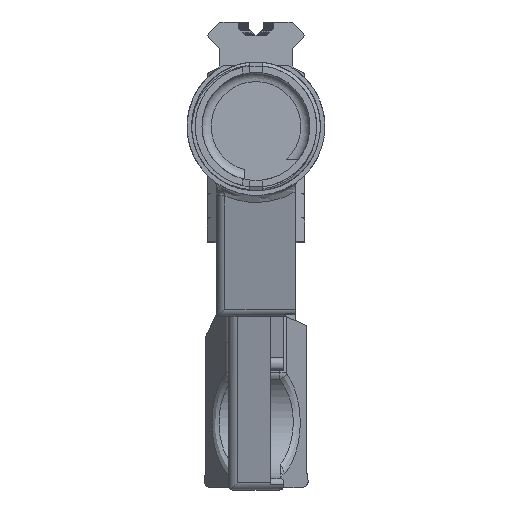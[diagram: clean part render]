
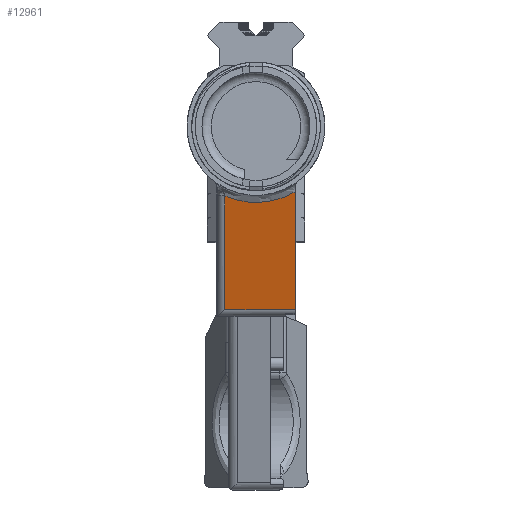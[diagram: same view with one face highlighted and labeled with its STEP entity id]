
A CAD part, front view. The second image highlights one B-rep face of the part: STEP entity #12961.
In plain terms, the highlighted planar face has unit normal (0, -0.972, -0.236).
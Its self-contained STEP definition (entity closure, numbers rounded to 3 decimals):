
#182=ELLIPSE('',#13804,17.416,16.925);
#598=PLANE('',#13806);
#1279=FACE_OUTER_BOUND('',#1988,.T.);
#1988=EDGE_LOOP('',(#11816,#11817,#11818,#11819));
#3605=LINE('',#23635,#4961);
#3606=LINE('',#23648,#4962);
#3612=LINE('',#23712,#4968);
#4961=VECTOR('',#16016,10.);
#4962=VECTOR('',#16019,10.);
#4968=VECTOR('',#16039,10.);
#6250=VERTEX_POINT('',#23632);
#6251=VERTEX_POINT('',#23634);
#6252=VERTEX_POINT('',#23647);
#6259=VERTEX_POINT('',#23707);
#7949=EDGE_CURVE('',#6250,#6251,#3605,.T.);
#7951=EDGE_CURVE('',#6251,#6252,#3606,.T.);
#7961=EDGE_CURVE('',#6259,#6250,#3612,.T.);
#8288=EDGE_CURVE('',#6252,#6259,#182,.T.);
#11816=ORIENTED_EDGE('',*,*,#7951,.F.);
#11817=ORIENTED_EDGE('',*,*,#7949,.F.);
#11818=ORIENTED_EDGE('',*,*,#7961,.F.);
#11819=ORIENTED_EDGE('',*,*,#8288,.F.);
#12961=ADVANCED_FACE('',(#1279),#598,.T.);
#13804=AXIS2_PLACEMENT_3D('',#25357,#16683,#16684);
#13806=AXIS2_PLACEMENT_3D('',#25375,#16687,#16688);
#16016=DIRECTION('',(-1.,0.,0.));
#16019=DIRECTION('',(0.,-0.236,0.972));
#16039=DIRECTION('',(0.,0.236,-0.972));
#16683=DIRECTION('center_axis',(0.,-0.972,
-0.236));
#16684=DIRECTION('ref_axis',(0.,0.236,-0.972));
#16687=DIRECTION('center_axis',(0.,-0.972,
-0.236));
#16688=DIRECTION('ref_axis',(0.,-0.236,0.972));
#23632=CARTESIAN_POINT('',(8.475,-63.716,1.529));
#23634=CARTESIAN_POINT('',(-6.725,-63.716,1.529));
#23635=CARTESIAN_POINT('',(7.25,-63.716,1.529));
#23647=CARTESIAN_POINT('',(-6.725,-69.681,26.122));
#23648=CARTESIAN_POINT('',(-6.725,-61.586,-7.255));
#23707=CARTESIAN_POINT('',(8.475,-69.895,27.003));
#23712=CARTESIAN_POINT('',(8.475,-70.017,27.507));
#25357=CARTESIAN_POINT('Origin',(0.,-73.449,
41.654));
#25375=CARTESIAN_POINT('Origin',(6.025,-63.346,0.));
